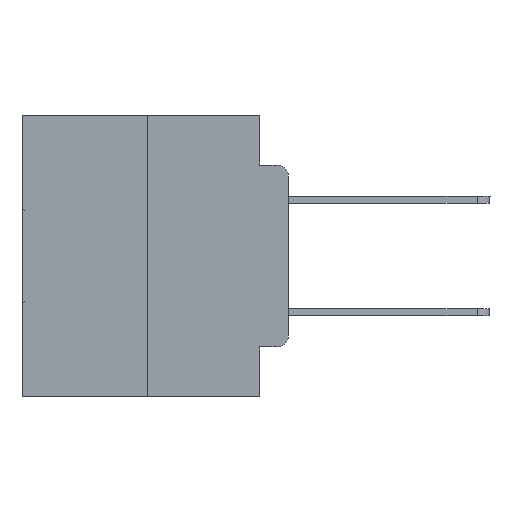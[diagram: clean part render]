
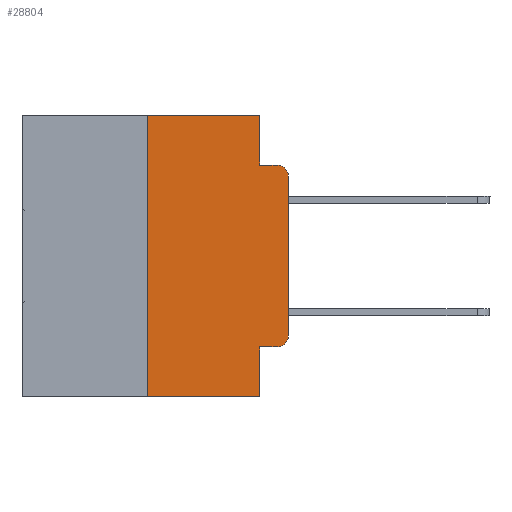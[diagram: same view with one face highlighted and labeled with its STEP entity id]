
A CAD part, left-side view. The second image highlights one B-rep face of the part: STEP entity #28804.
In plain terms, the highlighted planar face has unit normal (-1, 0, 0).
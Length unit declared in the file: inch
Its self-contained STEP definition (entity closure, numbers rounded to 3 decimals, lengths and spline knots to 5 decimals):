
#107 = AXIS2_PLACEMENT_3D ( 'NONE', #9609, #25962, #11922 ) ;
#592 = CARTESIAN_POINT ( 'NONE',  ( 0., 0.051, -0.0885 ) ) ;
#842 = LINE ( 'NONE', #17586, #12952 ) ;
#1447 = CARTESIAN_POINT ( 'NONE',  ( 0., 0.051, 0. ) ) ;
#2419 = VECTOR ( 'NONE', #28541, 39.37008 ) ;
#2457 = CARTESIAN_POINT ( 'NONE',  ( 0., 0.473, 0. ) ) ;
#3200 = VERTEX_POINT ( 'NONE', #20923 ) ;
#3790 = LINE ( 'NONE', #19981, #28190 ) ;
#3859 = EDGE_CURVE ( 'NONE', #5854, #25801, #23871, .T. ) ;
#3861 = VERTEX_POINT ( 'NONE', #18440 ) ;
#3926 = DIRECTION ( 'NONE',  ( 0., 0., -1. ) ) ;
#4253 = CARTESIAN_POINT ( 'NONE',  ( 0., 0.473, 0. ) ) ;
#4490 = CARTESIAN_POINT ( 'NONE',  ( 0., 0.25, 0. ) ) ;
#4572 = DIRECTION ( 'NONE',  ( 0., 0., 1. ) ) ;
#4660 = CARTESIAN_POINT ( 'NONE',  ( 0., 0.051, -0.4115 ) ) ;
#4679 = CARTESIAN_POINT ( 'NONE',  ( 0., 0., -0.3915 ) ) ;
#4737 = CARTESIAN_POINT ( 'NONE',  ( 0., 0.02, -0.1085 ) ) ;
#5197 = CIRCLE ( 'NONE', #107, 0.02 ) ;
#5531 = EDGE_CURVE ( 'NONE', #23548, #9098, #14185, .T. ) ;
#5738 = LINE ( 'NONE', #1447, #23826 ) ;
#5854 = VERTEX_POINT ( 'NONE', #9272 ) ;
#6009 = CARTESIAN_POINT ( 'NONE',  ( 0., 0., -0.1085 ) ) ;
#6661 = ORIENTED_EDGE ( 'NONE', *, *, #5531, .F. ) ;
#6843 = AXIS2_PLACEMENT_3D ( 'NONE', #4253, #25584, #11532 ) ;
#7028 = VECTOR ( 'NONE', #21298, 39.37008 ) ;
#7260 = DIRECTION ( 'NONE',  ( 0., 0., -1. ) ) ;
#7768 = ORIENTED_EDGE ( 'NONE', *, *, #16686, .T. ) ;
#7949 = VECTOR ( 'NONE', #26966, 39.37008 ) ;
#8173 = ORIENTED_EDGE ( 'NONE', *, *, #13374, .F. ) ;
#9098 = VERTEX_POINT ( 'NONE', #15564 ) ;
#9212 = PLANE ( 'NONE',  #6843 ) ;
#9246 = ORIENTED_EDGE ( 'NONE', *, *, #3859, .F. ) ;
#9272 = CARTESIAN_POINT ( 'NONE',  ( 0., 0.25, -0.5 ) ) ;
#9609 = CARTESIAN_POINT ( 'NONE',  ( 0., 0.02, -0.3915 ) ) ;
#9644 = EDGE_CURVE ( 'NONE', #5854, #25517, #842, .T. ) ;
#10526 = CARTESIAN_POINT ( 'NONE',  ( 0., 0.051, -0.5 ) ) ;
#10675 = ORIENTED_EDGE ( 'NONE', *, *, #22004, .F. ) ;
#10679 = VERTEX_POINT ( 'NONE', #4679 ) ;
#11532 = DIRECTION ( 'NONE',  ( 0., 0., -1. ) ) ;
#11922 = DIRECTION ( 'NONE',  ( 0., 0., -1. ) ) ;
#12137 = ORIENTED_EDGE ( 'NONE', *, *, #18864, .T. ) ;
#12173 = ORIENTED_EDGE ( 'NONE', *, *, #13514, .F. ) ;
#12952 = VECTOR ( 'NONE', #15206, 39.37008 ) ;
#13265 = LINE ( 'NONE', #4660, #7028 ) ;
#13374 = EDGE_CURVE ( 'NONE', #25801, #23548, #15930, .T. ) ;
#13514 = EDGE_CURVE ( 'NONE', #9098, #3861, #23993, .T. ) ;
#13758 = FACE_OUTER_BOUND ( 'NONE', #24239, .T. ) ;
#14185 = LINE ( 'NONE', #29316, #7949 ) ;
#15034 = DIRECTION ( 'NONE',  ( 0., -1., 0. ) ) ;
#15036 = VERTEX_POINT ( 'NONE', #18793 ) ;
#15079 = EDGE_CURVE ( 'NONE', #23591, #3861, #23230, .T. ) ;
#15206 = DIRECTION ( 'NONE',  ( 0., -1., 0. ) ) ;
#15564 = CARTESIAN_POINT ( 'NONE',  ( 0., 0.051, -0.0885 ) ) ;
#15930 = LINE ( 'NONE', #2457, #2419 ) ;
#16487 = CARTESIAN_POINT ( 'NONE',  ( 0., 0.25, 0. ) ) ;
#16686 = EDGE_CURVE ( 'NONE', #10679, #23591, #3790, .T. ) ;
#17586 = CARTESIAN_POINT ( 'NONE',  ( 0., 0.473, -0.5 ) ) ;
#18392 = VECTOR ( 'NONE', #4572, 39.37008 ) ;
#18440 = CARTESIAN_POINT ( 'NONE',  ( 0., 0.02, -0.0885 ) ) ;
#18793 = CARTESIAN_POINT ( 'NONE',  ( 0., 0.02, -0.4115 ) ) ;
#18864 = EDGE_CURVE ( 'NONE', #15036, #10679, #5197, .T. ) ;
#19205 = AXIS2_PLACEMENT_3D ( 'NONE', #4737, #21354, #7260 ) ;
#19981 = CARTESIAN_POINT ( 'NONE',  ( 0., 0., 0. ) ) ;
#20425 = EDGE_CURVE ( 'NONE', #3200, #15036, #13265, .T. ) ;
#20923 = CARTESIAN_POINT ( 'NONE',  ( 0., 0.051, -0.4115 ) ) ;
#21298 = DIRECTION ( 'NONE',  ( 0., -1., 0. ) ) ;
#21354 = DIRECTION ( 'NONE',  ( -1., 0., 0. ) ) ;
#21722 = ORIENTED_EDGE ( 'NONE', *, *, #9644, .T. ) ;
#22004 = EDGE_CURVE ( 'NONE', #3200, #25517, #5738, .T. ) ;
#22326 = CARTESIAN_POINT ( 'NONE',  ( 0., 0.051, 0. ) ) ;
#22447 = DIRECTION ( 'NONE',  ( 0., 0., 1. ) ) ;
#23230 = CIRCLE ( 'NONE', #19205, 0.02 ) ;
#23548 = VERTEX_POINT ( 'NONE', #22326 ) ;
#23591 = VERTEX_POINT ( 'NONE', #6009 ) ;
#23826 = VECTOR ( 'NONE', #3926, 39.37008 ) ;
#23871 = LINE ( 'NONE', #4490, #18392 ) ;
#23993 = LINE ( 'NONE', #592, #29449 ) ;
#24239 = EDGE_LOOP ( 'NONE', ( #7768, #26468, #12173, #6661, #8173, #9246, #21722, #10675, #30104, #12137 ) ) ;
#25517 = VERTEX_POINT ( 'NONE', #10526 ) ;
#25584 = DIRECTION ( 'NONE',  ( 1., 0., 0. ) ) ;
#25801 = VERTEX_POINT ( 'NONE', #16487 ) ;
#25962 = DIRECTION ( 'NONE',  ( -1., 0., 0. ) ) ;
#26468 = ORIENTED_EDGE ( 'NONE', *, *, #15079, .T. ) ;
#26966 = DIRECTION ( 'NONE',  ( 0., 0., -1. ) ) ;
#28190 = VECTOR ( 'NONE', #22447, 39.37008 ) ;
#28541 = DIRECTION ( 'NONE',  ( 0., -1., 0. ) ) ;
#28804 = ADVANCED_FACE ( 'NONE', ( #13758 ), #9212, .F. ) ;
#29316 = CARTESIAN_POINT ( 'NONE',  ( 0., 0.051, 0. ) ) ;
#29449 = VECTOR ( 'NONE', #15034, 39.37008 ) ;
#30104 = ORIENTED_EDGE ( 'NONE', *, *, #20425, .T. ) ;
